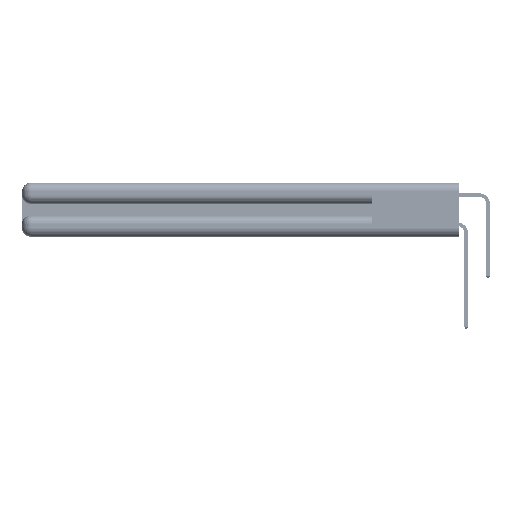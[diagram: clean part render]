
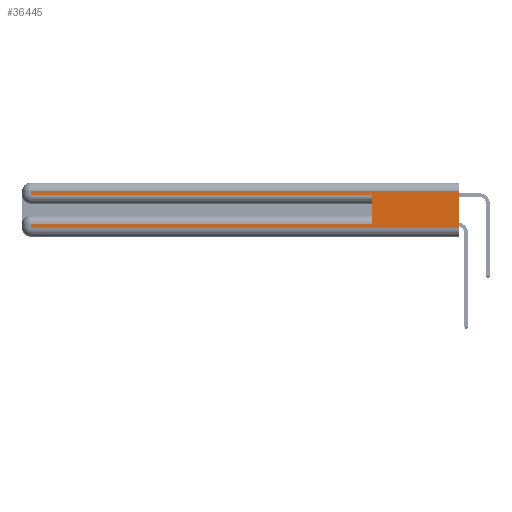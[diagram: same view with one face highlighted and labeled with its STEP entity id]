
A CAD part, left-side view. The second image highlights one B-rep face of the part: STEP entity #36445.
In plain terms, the highlighted planar face has unit normal (-1, 0, 0).
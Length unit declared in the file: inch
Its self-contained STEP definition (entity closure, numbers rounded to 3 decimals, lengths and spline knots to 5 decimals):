
#472 = VERTEX_POINT ( 'NONE', #9034 ) ;
#753 = CARTESIAN_POINT ( 'NONE',  ( 0., 0., 0.31 ) ) ;
#971 = LINE ( 'NONE', #39445, #12414 ) ;
#1592 = CARTESIAN_POINT ( 'NONE',  ( 0., 0., 0.06 ) ) ;
#2838 = VECTOR ( 'NONE', #13664, 39.37008 ) ;
#3028 = EDGE_CURVE ( 'NONE', #472, #20313, #54914, .T. ) ;
#3255 = VECTOR ( 'NONE', #18258, 39.37008 ) ;
#3602 = AXIS2_PLACEMENT_3D ( 'NONE', #15034, #36907, #11119 ) ;
#4477 = ORIENTED_EDGE ( 'NONE', *, *, #40300, .F. ) ;
#5582 = VERTEX_POINT ( 'NONE', #20743 ) ;
#6027 = VECTOR ( 'NONE', #24649, 39.37008 ) ;
#7301 = EDGE_LOOP ( 'NONE', ( #21827, #9750, #25088, #29026, #4477, #24300, #29779, #49537 ) ) ;
#7455 = CARTESIAN_POINT ( 'NONE',  ( 0., 0.6, 0.085 ) ) ;
#7704 = VERTEX_POINT ( 'NONE', #8518 ) ;
#7909 = CARTESIAN_POINT ( 'NONE',  ( 0., 0.6, 0.145 ) ) ;
#8198 = DIRECTION ( 'NONE',  ( 0., -1., 0. ) ) ;
#8271 = DIRECTION ( 'NONE',  ( 0., 0., 1. ) ) ;
#8518 = CARTESIAN_POINT ( 'NONE',  ( 0., 0.6, 0.285 ) ) ;
#9034 = CARTESIAN_POINT ( 'NONE',  ( 0., 2.94, 0.06 ) ) ;
#9693 = CARTESIAN_POINT ( 'NONE',  ( 0., 0., 0.31 ) ) ;
#9750 = ORIENTED_EDGE ( 'NONE', *, *, #55023, .T. ) ;
#11119 = DIRECTION ( 'NONE',  ( 0., 0., -1. ) ) ;
#12414 = VECTOR ( 'NONE', #30997, 39.37008 ) ;
#12975 = EDGE_CURVE ( 'NONE', #21641, #49879, #18721, .T. ) ;
#13664 = DIRECTION ( 'NONE',  ( 0., 0., -1. ) ) ;
#14302 = LINE ( 'NONE', #22439, #2838 ) ;
#15034 = CARTESIAN_POINT ( 'NONE',  ( 0., 0., 0.37 ) ) ;
#15395 = EDGE_CURVE ( 'NONE', #26038, #20313, #18769, .T. ) ;
#18258 = DIRECTION ( 'NONE',  ( 0., 1., 0. ) ) ;
#18721 = LINE ( 'NONE', #42723, #24717 ) ;
#18759 = CARTESIAN_POINT ( 'NONE',  ( 0., 2.94, 0.285 ) ) ;
#18769 = LINE ( 'NONE', #20388, #6027 ) ;
#20313 = VERTEX_POINT ( 'NONE', #45707 ) ;
#20388 = CARTESIAN_POINT ( 'NONE',  ( 0., 0., 0.37 ) ) ;
#20743 = CARTESIAN_POINT ( 'NONE',  ( 0., 2.94, 0.31 ) ) ;
#21641 = VERTEX_POINT ( 'NONE', #7455 ) ;
#21827 = ORIENTED_EDGE ( 'NONE', *, *, #15395, .F. ) ;
#22439 = CARTESIAN_POINT ( 'NONE',  ( 0., 2.94, 0.37 ) ) ;
#23386 = CARTESIAN_POINT ( 'NONE',  ( 0., 2.94, 0.085 ) ) ;
#24300 = ORIENTED_EDGE ( 'NONE', *, *, #12975, .T. ) ;
#24649 = DIRECTION ( 'NONE',  ( 0., 0., -1. ) ) ;
#24717 = VECTOR ( 'NONE', #34285, 39.37008 ) ;
#25088 = ORIENTED_EDGE ( 'NONE', *, *, #25478, .T. ) ;
#25478 = EDGE_CURVE ( 'NONE', #5582, #32630, #971, .T. ) ;
#26038 = VERTEX_POINT ( 'NONE', #753 ) ;
#27012 = EDGE_CURVE ( 'NONE', #32630, #7704, #34906, .T. ) ;
#29026 = ORIENTED_EDGE ( 'NONE', *, *, #27012, .T. ) ;
#29779 = ORIENTED_EDGE ( 'NONE', *, *, #45688, .T. ) ;
#30997 = DIRECTION ( 'NONE',  ( 0., 0., -1. ) ) ;
#32630 = VERTEX_POINT ( 'NONE', #18759 ) ;
#34285 = DIRECTION ( 'NONE',  ( 0., 1., 0. ) ) ;
#34906 = LINE ( 'NONE', #49574, #40959 ) ;
#35709 = VECTOR ( 'NONE', #8271, 39.37008 ) ;
#36445 = ADVANCED_FACE ( 'NONE', ( #40086 ), #49034, .F. ) ;
#36907 = DIRECTION ( 'NONE',  ( 1., 0., 0. ) ) ;
#39445 = CARTESIAN_POINT ( 'NONE',  ( 0., 2.94, 0.37 ) ) ;
#40086 = FACE_OUTER_BOUND ( 'NONE', #7301, .T. ) ;
#40300 = EDGE_CURVE ( 'NONE', #21641, #7704, #49759, .T. ) ;
#40959 = VECTOR ( 'NONE', #8198, 39.37008 ) ;
#41492 = LINE ( 'NONE', #9693, #3255 ) ;
#42723 = CARTESIAN_POINT ( 'NONE',  ( 0., 0., 0.085 ) ) ;
#45688 = EDGE_CURVE ( 'NONE', #49879, #472, #14302, .T. ) ;
#45707 = CARTESIAN_POINT ( 'NONE',  ( 0., 0., 0.06 ) ) ;
#48784 = DIRECTION ( 'NONE',  ( 0., -1., 0. ) ) ;
#49034 = PLANE ( 'NONE',  #3602 ) ;
#49537 = ORIENTED_EDGE ( 'NONE', *, *, #3028, .T. ) ;
#49574 = CARTESIAN_POINT ( 'NONE',  ( 0., 0., 0.285 ) ) ;
#49759 = LINE ( 'NONE', #7909, #35709 ) ;
#49879 = VERTEX_POINT ( 'NONE', #23386 ) ;
#50290 = VECTOR ( 'NONE', #48784, 39.37008 ) ;
#54914 = LINE ( 'NONE', #1592, #50290 ) ;
#55023 = EDGE_CURVE ( 'NONE', #26038, #5582, #41492, .T. ) ;
